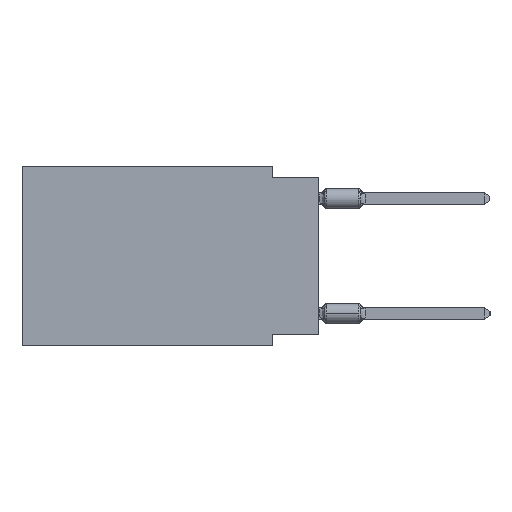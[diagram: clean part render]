
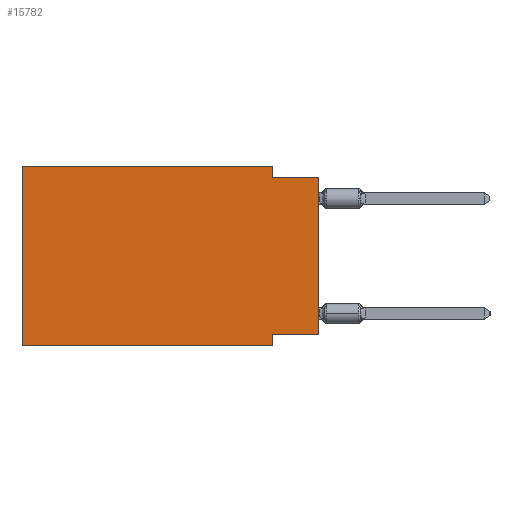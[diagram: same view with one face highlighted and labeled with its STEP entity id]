
A CAD part, left-side view. The second image highlights one B-rep face of the part: STEP entity #15782.
In plain terms, the highlighted planar face has unit normal (-1, 0, 0).
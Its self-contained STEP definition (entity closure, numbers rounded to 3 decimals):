
#448 = LINE ( 'NONE', #16289, #2022 ) ;
#859 = LINE ( 'NONE', #21839, #22057 ) ;
#2022 = VECTOR ( 'NONE', #26769, 1000. ) ;
#2050 = EDGE_CURVE ( 'NONE', #11731, #12311, #448, .T. ) ;
#2736 = VECTOR ( 'NONE', #30803, 1000. ) ;
#3436 = VERTEX_POINT ( 'NONE', #10442 ) ;
#3794 = AXIS2_PLACEMENT_3D ( 'NONE', #10263, #5100, #23496 ) ;
#3836 = ORIENTED_EDGE ( 'NONE', *, *, #23523, .F. ) ;
#3981 = DIRECTION ( 'NONE',  ( 0., 0., 1. ) ) ;
#4040 = CARTESIAN_POINT ( 'NONE',  ( 0., 16.383, -9.906 ) ) ;
#5100 = DIRECTION ( 'NONE',  ( 1., 0., 0. ) ) ;
#5698 = ORIENTED_EDGE ( 'NONE', *, *, #24381, .T. ) ;
#6088 = VERTEX_POINT ( 'NONE', #11497 ) ;
#6966 = LINE ( 'NONE', #4040, #28179 ) ;
#7895 = CARTESIAN_POINT ( 'NONE',  ( 0., 2.54, 0. ) ) ;
#8682 = EDGE_CURVE ( 'NONE', #6088, #9315, #859, .T. ) ;
#8959 = EDGE_CURVE ( 'NONE', #18625, #13645, #26621, .T. ) ;
#9315 = VERTEX_POINT ( 'NONE', #29623 ) ;
#9463 = VECTOR ( 'NONE', #13058, 1000. ) ;
#10110 = EDGE_CURVE ( 'NONE', #6088, #13645, #6966, .T. ) ;
#10263 = CARTESIAN_POINT ( 'NONE',  ( 0., 16.383, 0. ) ) ;
#10442 = CARTESIAN_POINT ( 'NONE',  ( 0., 2.54, 0. ) ) ;
#10922 = CARTESIAN_POINT ( 'NONE',  ( 0., 0., -0.635 ) ) ;
#11388 = VECTOR ( 'NONE', #29420, 1000. ) ;
#11497 = CARTESIAN_POINT ( 'NONE',  ( 0., 16.383, -9.906 ) ) ;
#11731 = VERTEX_POINT ( 'NONE', #21834 ) ;
#11897 = CARTESIAN_POINT ( 'NONE',  ( 0., 0., 0. ) ) ;
#12311 = VERTEX_POINT ( 'NONE', #10922 ) ;
#12432 = CARTESIAN_POINT ( 'NONE',  ( 0., 16.383, 0. ) ) ;
#13058 = DIRECTION ( 'NONE',  ( 0., 0., -1. ) ) ;
#13645 = VERTEX_POINT ( 'NONE', #28308 ) ;
#14598 = DIRECTION ( 'NONE',  ( 0., 0., -1. ) ) ;
#15242 = ORIENTED_EDGE ( 'NONE', *, *, #16588, .F. ) ;
#15417 = FACE_OUTER_BOUND ( 'NONE', #30196, .T. ) ;
#15782 = ADVANCED_FACE ( 'NONE', ( #15417 ), #23325, .F. ) ;
#15965 = CARTESIAN_POINT ( 'NONE',  ( 0., 2.54, -9.906 ) ) ;
#16289 = CARTESIAN_POINT ( 'NONE',  ( 0., 0., -0.635 ) ) ;
#16526 = EDGE_CURVE ( 'NONE', #9315, #3436, #25481, .T. ) ;
#16588 = EDGE_CURVE ( 'NONE', #26030, #18625, #18929, .T. ) ;
#16613 = VECTOR ( 'NONE', #3981, 1000. ) ;
#18295 = ORIENTED_EDGE ( 'NONE', *, *, #10110, .T. ) ;
#18625 = VERTEX_POINT ( 'NONE', #33623 ) ;
#18929 = LINE ( 'NONE', #24241, #11388 ) ;
#20097 = VECTOR ( 'NONE', #14598, 1000. ) ;
#21488 = ORIENTED_EDGE ( 'NONE', *, *, #16526, .F. ) ;
#21834 = CARTESIAN_POINT ( 'NONE',  ( 0., 2.54, -0.635 ) ) ;
#21839 = CARTESIAN_POINT ( 'NONE',  ( 0., 16.383, 0. ) ) ;
#22057 = VECTOR ( 'NONE', #27169, 1000. ) ;
#22544 = ORIENTED_EDGE ( 'NONE', *, *, #2050, .F. ) ;
#23032 = ORIENTED_EDGE ( 'NONE', *, *, #8682, .F. ) ;
#23325 = PLANE ( 'NONE',  #3794 ) ;
#23496 = DIRECTION ( 'NONE',  ( 0., 0., -1. ) ) ;
#23523 = EDGE_CURVE ( 'NONE', #3436, #11731, #26811, .T. ) ;
#24241 = CARTESIAN_POINT ( 'NONE',  ( 0., 0., -9.271 ) ) ;
#24381 = EDGE_CURVE ( 'NONE', #26030, #12311, #30629, .T. ) ;
#25481 = LINE ( 'NONE', #12432, #2736 ) ;
#26030 = VERTEX_POINT ( 'NONE', #31097 ) ;
#26621 = LINE ( 'NONE', #15965, #9463 ) ;
#26769 = DIRECTION ( 'NONE',  ( 0., -1., 0. ) ) ;
#26811 = LINE ( 'NONE', #7895, #20097 ) ;
#27169 = DIRECTION ( 'NONE',  ( 0., 0., 1. ) ) ;
#27930 = ORIENTED_EDGE ( 'NONE', *, *, #8959, .F. ) ;
#28179 = VECTOR ( 'NONE', #30180, 1000. ) ;
#28308 = CARTESIAN_POINT ( 'NONE',  ( 0., 2.54, -9.906 ) ) ;
#29420 = DIRECTION ( 'NONE',  ( 0., 1., 0. ) ) ;
#29623 = CARTESIAN_POINT ( 'NONE',  ( 0., 16.383, 0. ) ) ;
#30180 = DIRECTION ( 'NONE',  ( 0., -1., 0. ) ) ;
#30196 = EDGE_LOOP ( 'NONE', ( #5698, #22544, #3836, #21488, #23032, #18295, #27930, #15242 ) ) ;
#30629 = LINE ( 'NONE', #11897, #16613 ) ;
#30803 = DIRECTION ( 'NONE',  ( 0., -1., 0. ) ) ;
#31097 = CARTESIAN_POINT ( 'NONE',  ( 0., 0., -9.271 ) ) ;
#33623 = CARTESIAN_POINT ( 'NONE',  ( 0., 2.54, -9.271 ) ) ;
